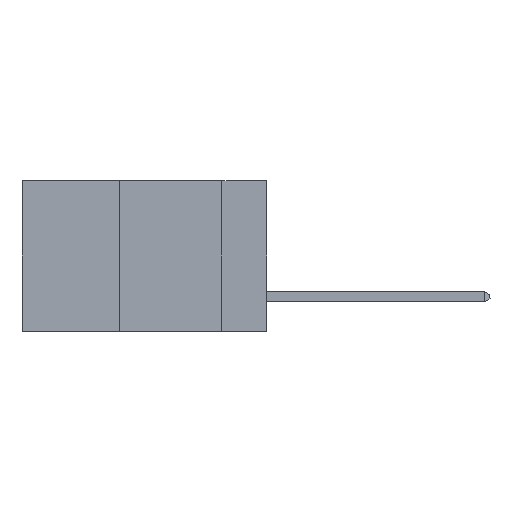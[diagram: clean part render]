
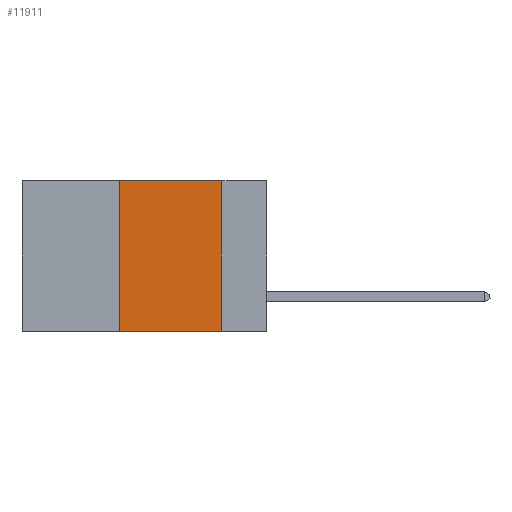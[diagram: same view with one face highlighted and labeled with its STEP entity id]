
A CAD part, left-side view. The second image highlights one B-rep face of the part: STEP entity #11911.
In plain terms, the highlighted planar face has unit normal (-1, 0, 0).
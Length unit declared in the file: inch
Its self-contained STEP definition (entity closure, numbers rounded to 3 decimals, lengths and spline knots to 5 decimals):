
#936 = VECTOR ( 'NONE', #17095, 39.37008 ) ;
#1772 = VERTEX_POINT ( 'NONE', #15074 ) ;
#1865 = ORIENTED_EDGE ( 'NONE', *, *, #9557, .T. ) ;
#2151 = CARTESIAN_POINT ( 'NONE',  ( 0., 0.11, -0.37 ) ) ;
#2628 = AXIS2_PLACEMENT_3D ( 'NONE', #12418, #4045, #13786 ) ;
#3257 = CARTESIAN_POINT ( 'NONE',  ( 0., 0.11, 0. ) ) ;
#3433 = LINE ( 'NONE', #5018, #10484 ) ;
#4045 = DIRECTION ( 'NONE',  ( 1., 0., 0. ) ) ;
#5018 = CARTESIAN_POINT ( 'NONE',  ( 0., 0.6, -0.37 ) ) ;
#5238 = ORIENTED_EDGE ( 'NONE', *, *, #15353, .F. ) ;
#5279 = LINE ( 'NONE', #3257, #936 ) ;
#5349 = VECTOR ( 'NONE', #8594, 39.37008 ) ;
#6533 = CARTESIAN_POINT ( 'NONE',  ( 0., 0.36, -0.37 ) ) ;
#6853 = VERTEX_POINT ( 'NONE', #6533 ) ;
#7183 = CARTESIAN_POINT ( 'NONE',  ( 0., 0.6, 0. ) ) ;
#7855 = VECTOR ( 'NONE', #15918, 39.37008 ) ;
#8564 = ORIENTED_EDGE ( 'NONE', *, *, #17601, .F. ) ;
#8594 = DIRECTION ( 'NONE',  ( 0., -1., 0. ) ) ;
#8940 = VERTEX_POINT ( 'NONE', #2151 ) ;
#9094 = CARTESIAN_POINT ( 'NONE',  ( 0., 0.36, 0. ) ) ;
#9557 = EDGE_CURVE ( 'NONE', #6853, #8940, #3433, .T. ) ;
#10133 = EDGE_CURVE ( 'NONE', #6853, #1772, #11947, .T. ) ;
#10413 = FACE_OUTER_BOUND ( 'NONE', #10771, .T. ) ;
#10484 = VECTOR ( 'NONE', #13337, 39.37008 ) ;
#10771 = EDGE_LOOP ( 'NONE', ( #8564, #5238, #12650, #1865 ) ) ;
#11911 = ADVANCED_FACE ( 'NONE', ( #10413 ), #16426, .F. ) ;
#11947 = LINE ( 'NONE', #9094, #7855 ) ;
#12418 = CARTESIAN_POINT ( 'NONE',  ( 0., 0.6, 0. ) ) ;
#12650 = ORIENTED_EDGE ( 'NONE', *, *, #10133, .F. ) ;
#13070 = VERTEX_POINT ( 'NONE', #15063 ) ;
#13337 = DIRECTION ( 'NONE',  ( 0., -1., 0. ) ) ;
#13786 = DIRECTION ( 'NONE',  ( 0., 0., -1. ) ) ;
#15063 = CARTESIAN_POINT ( 'NONE',  ( 0., 0.11, 0. ) ) ;
#15074 = CARTESIAN_POINT ( 'NONE',  ( 0., 0.36, 0. ) ) ;
#15353 = EDGE_CURVE ( 'NONE', #1772, #13070, #16747, .T. ) ;
#15918 = DIRECTION ( 'NONE',  ( 0., 0., 1. ) ) ;
#16426 = PLANE ( 'NONE',  #2628 ) ;
#16747 = LINE ( 'NONE', #7183, #5349 ) ;
#17095 = DIRECTION ( 'NONE',  ( 0., 0., -1. ) ) ;
#17601 = EDGE_CURVE ( 'NONE', #13070, #8940, #5279, .T. ) ;
